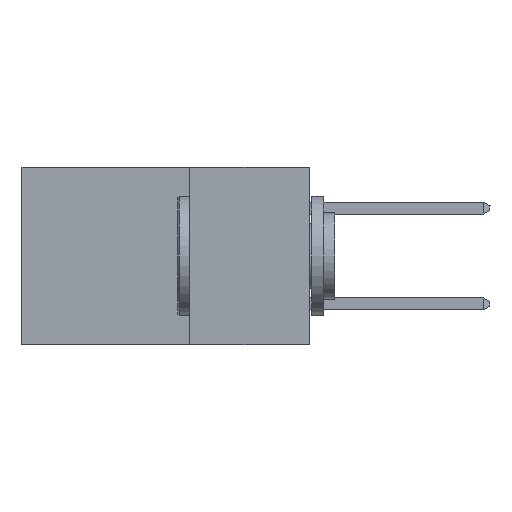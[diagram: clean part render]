
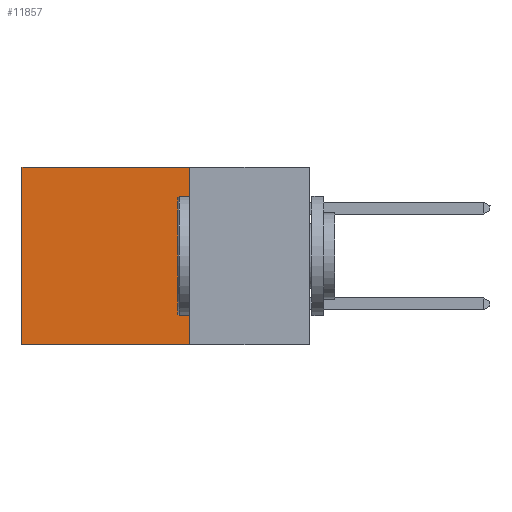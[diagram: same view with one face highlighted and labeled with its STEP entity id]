
A CAD part, left-side view. The second image highlights one B-rep face of the part: STEP entity #11857.
In plain terms, the highlighted planar face has unit normal (-1, 0, 0).
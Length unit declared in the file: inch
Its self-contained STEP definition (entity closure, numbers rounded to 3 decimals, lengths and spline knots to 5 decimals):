
#1892 = LINE ( 'NONE', #16195, #5229 ) ;
#2035 = CARTESIAN_POINT ( 'NONE',  ( 0.2875, 0.6, 0. ) ) ;
#2793 = DIRECTION ( 'NONE',  ( 0., 0., -1. ) ) ;
#3285 = CARTESIAN_POINT ( 'NONE',  ( 0.2875, 0.25, 0. ) ) ;
#3312 = VERTEX_POINT ( 'NONE', #8071 ) ;
#3843 = LINE ( 'NONE', #3889, #7821 ) ;
#3889 = CARTESIAN_POINT ( 'NONE',  ( 0.2875, 0.25, 0. ) ) ;
#4286 = EDGE_CURVE ( 'NONE', #13684, #6524, #15069, .T. ) ;
#4376 = AXIS2_PLACEMENT_3D ( 'NONE', #3285, #16624, #11102 ) ;
#5229 = VECTOR ( 'NONE', #6833, 39.37008 ) ;
#5534 = ORIENTED_EDGE ( 'NONE', *, *, #13806, .T. ) ;
#6524 = VERTEX_POINT ( 'NONE', #17251 ) ;
#6728 = FACE_OUTER_BOUND ( 'NONE', #7078, .T. ) ;
#6833 = DIRECTION ( 'NONE',  ( 0., 1., 0. ) ) ;
#7034 = CARTESIAN_POINT ( 'NONE',  ( 0.2875, 0.6, 0. ) ) ;
#7078 = EDGE_LOOP ( 'NONE', ( #5534, #11188, #16134, #9204 ) ) ;
#7520 = VECTOR ( 'NONE', #16740, 39.37008 ) ;
#7821 = VECTOR ( 'NONE', #2793, 39.37008 ) ;
#8071 = CARTESIAN_POINT ( 'NONE',  ( 0.2875, 0.25, 0. ) ) ;
#8181 = CARTESIAN_POINT ( 'NONE',  ( 0.2875, 0.25, -0.37 ) ) ;
#8832 = EDGE_CURVE ( 'NONE', #3312, #15113, #1892, .T. ) ;
#9204 = ORIENTED_EDGE ( 'NONE', *, *, #8832, .T. ) ;
#9578 = CARTESIAN_POINT ( 'NONE',  ( 0.2875, 0.25, -0.37 ) ) ;
#11102 = DIRECTION ( 'NONE',  ( 0., 0., -1. ) ) ;
#11188 = ORIENTED_EDGE ( 'NONE', *, *, #4286, .F. ) ;
#11269 = PLANE ( 'NONE',  #4376 ) ;
#11857 = ADVANCED_FACE ( 'NONE', ( #6728 ), #11269, .F. ) ;
#13684 = VERTEX_POINT ( 'NONE', #8181 ) ;
#13806 = EDGE_CURVE ( 'NONE', #15113, #6524, #15512, .T. ) ;
#14915 = DIRECTION ( 'NONE',  ( 0., 1., 0. ) ) ;
#15069 = LINE ( 'NONE', #9578, #16524 ) ;
#15113 = VERTEX_POINT ( 'NONE', #2035 ) ;
#15512 = LINE ( 'NONE', #7034, #7520 ) ;
#16108 = EDGE_CURVE ( 'NONE', #3312, #13684, #3843, .T. ) ;
#16134 = ORIENTED_EDGE ( 'NONE', *, *, #16108, .F. ) ;
#16195 = CARTESIAN_POINT ( 'NONE',  ( 0.2875, 0.25, 0. ) ) ;
#16524 = VECTOR ( 'NONE', #14915, 39.37008 ) ;
#16624 = DIRECTION ( 'NONE',  ( 1., 0., 0. ) ) ;
#16740 = DIRECTION ( 'NONE',  ( 0., 0., -1. ) ) ;
#17251 = CARTESIAN_POINT ( 'NONE',  ( 0.2875, 0.6, -0.37 ) ) ;
